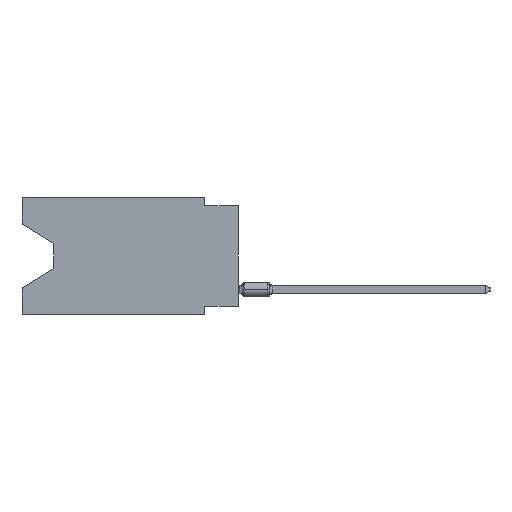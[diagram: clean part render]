
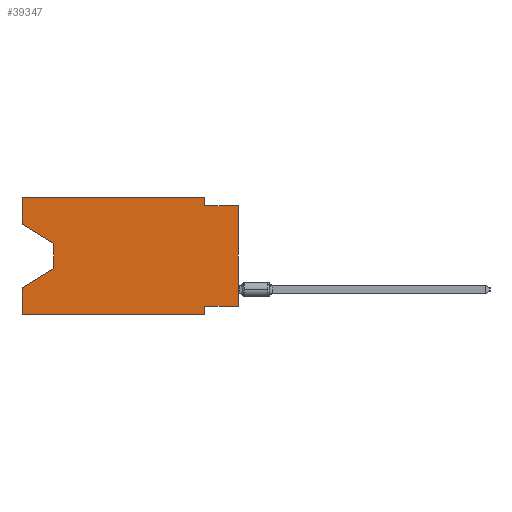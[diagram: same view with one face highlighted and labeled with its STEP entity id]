
A CAD part, left-side view. The second image highlights one B-rep face of the part: STEP entity #39347.
In plain terms, the highlighted planar face has unit normal (-1, 0, 0).
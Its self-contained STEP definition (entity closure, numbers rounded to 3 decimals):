
#670 = LINE ( 'NONE', #19186, #1400 ) ;
#745 = VECTOR ( 'NONE', #2986, 1000. ) ;
#812 = VERTEX_POINT ( 'NONE', #41530 ) ;
#1118 = ORIENTED_EDGE ( 'NONE', *, *, #11759, .T. ) ;
#1400 = VECTOR ( 'NONE', #22766, 1000. ) ;
#2557 = CARTESIAN_POINT ( 'NONE',  ( 0., 2.54, 0. ) ) ;
#2986 = DIRECTION ( 'NONE',  ( 0., 0., 1. ) ) ;
#3231 = CARTESIAN_POINT ( 'NONE',  ( 0., 0., 0. ) ) ;
#3430 = VECTOR ( 'NONE', #35877, 1000. ) ;
#3504 = ORIENTED_EDGE ( 'NONE', *, *, #15011, .T. ) ;
#3566 = VERTEX_POINT ( 'NONE', #45444 ) ;
#5263 = CARTESIAN_POINT ( 'NONE',  ( 0., 16.383, 0. ) ) ;
#5274 = VERTEX_POINT ( 'NONE', #5263 ) ;
#5816 = ORIENTED_EDGE ( 'NONE', *, *, #46398, .F. ) ;
#6011 = ORIENTED_EDGE ( 'NONE', *, *, #12647, .T. ) ;
#6491 = EDGE_CURVE ( 'NONE', #15405, #45929, #42858, .T. ) ;
#6993 = LINE ( 'NONE', #28385, #12425 ) ;
#7243 = LINE ( 'NONE', #25737, #43399 ) ;
#7698 = EDGE_CURVE ( 'NONE', #36288, #3566, #29592, .T. ) ;
#8846 = CARTESIAN_POINT ( 'NONE',  ( 0., 16.383, 0. ) ) ;
#9758 = LINE ( 'NONE', #2557, #27354 ) ;
#10437 = EDGE_CURVE ( 'NONE', #45929, #31728, #40064, .T. ) ;
#10516 = VERTEX_POINT ( 'NONE', #29495 ) ;
#11190 = VECTOR ( 'NONE', #22400, 1000. ) ;
#11759 = EDGE_CURVE ( 'NONE', #15405, #44175, #46711, .T. ) ;
#12163 = VECTOR ( 'NONE', #35338, 1000. ) ;
#12425 = VECTOR ( 'NONE', #20703, 1000. ) ;
#12647 = EDGE_CURVE ( 'NONE', #36288, #31728, #14582, .T. ) ;
#13265 = ORIENTED_EDGE ( 'NONE', *, *, #13916, .F. ) ;
#13916 = EDGE_CURVE ( 'NONE', #23383, #5274, #29414, .T. ) ;
#14513 = VERTEX_POINT ( 'NONE', #23809 ) ;
#14582 = LINE ( 'NONE', #33090, #31527 ) ;
#15011 = EDGE_CURVE ( 'NONE', #14513, #3566, #37028, .T. ) ;
#15405 = VERTEX_POINT ( 'NONE', #15971 ) ;
#15971 = CARTESIAN_POINT ( 'NONE',  ( 0., 0., -8.255 ) ) ;
#16225 = EDGE_CURVE ( 'NONE', #812, #44175, #670, .T. ) ;
#19186 = CARTESIAN_POINT ( 'NONE',  ( 0., 0., -0.635 ) ) ;
#19281 = CARTESIAN_POINT ( 'NONE',  ( 0., 2.54, 0. ) ) ;
#19666 = FACE_OUTER_BOUND ( 'NONE', #25329, .T. ) ;
#20646 = EDGE_CURVE ( 'NONE', #5274, #33728, #27756, .T. ) ;
#20703 = DIRECTION ( 'NONE',  ( 0., 0., -1. ) ) ;
#21094 = ORIENTED_EDGE ( 'NONE', *, *, #10437, .F. ) ;
#22118 = ORIENTED_EDGE ( 'NONE', *, *, #31734, .T. ) ;
#22400 = DIRECTION ( 'NONE',  ( 0., 0., 1. ) ) ;
#22766 = DIRECTION ( 'NONE',  ( 0., -1., 0. ) ) ;
#22799 = CARTESIAN_POINT ( 'NONE',  ( 0., 16.383, -8.89 ) ) ;
#23043 = VECTOR ( 'NONE', #42412, 1000. ) ;
#23383 = VERTEX_POINT ( 'NONE', #42992 ) ;
#23809 = CARTESIAN_POINT ( 'NONE',  ( 0., 13.97, -5.385 ) ) ;
#24850 = CARTESIAN_POINT ( 'NONE',  ( 0., 0., -8.255 ) ) ;
#25329 = EDGE_LOOP ( 'NONE', ( #22118, #37161, #3504, #45902, #6011, #21094, #42938, #1118, #45962, #5816, #39247, #13265 ) ) ;
#25737 = CARTESIAN_POINT ( 'NONE',  ( 0., 16.383, -2.038 ) ) ;
#25791 = CARTESIAN_POINT ( 'NONE',  ( 0., 16.383, 0. ) ) ;
#26452 = CARTESIAN_POINT ( 'NONE',  ( 0., 13.97, -5.385 ) ) ;
#27354 = VECTOR ( 'NONE', #27809, 1000. ) ;
#27397 = VECTOR ( 'NONE', #37972, 1000. ) ;
#27425 = CARTESIAN_POINT ( 'NONE',  ( 0., 0., -0.635 ) ) ;
#27655 = DIRECTION ( 'NONE',  ( 0., -1., 0. ) ) ;
#27756 = LINE ( 'NONE', #34939, #23043 ) ;
#27809 = DIRECTION ( 'NONE',  ( 0., 0., -1. ) ) ;
#28018 = EDGE_CURVE ( 'NONE', #10516, #14513, #6993, .T. ) ;
#28385 = CARTESIAN_POINT ( 'NONE',  ( 0., 13.97, -3.505 ) ) ;
#29414 = LINE ( 'NONE', #25791, #33573 ) ;
#29495 = CARTESIAN_POINT ( 'NONE',  ( 0., 13.97, -3.505 ) ) ;
#29592 = LINE ( 'NONE', #33682, #11190 ) ;
#31527 = VECTOR ( 'NONE', #27655, 1000. ) ;
#31728 = VERTEX_POINT ( 'NONE', #43504 ) ;
#31734 = EDGE_CURVE ( 'NONE', #23383, #10516, #7243, .T. ) ;
#32162 = CARTESIAN_POINT ( 'NONE',  ( 0., 2.54, -8.255 ) ) ;
#33090 = CARTESIAN_POINT ( 'NONE',  ( 0., 16.383, -8.89 ) ) ;
#33573 = VECTOR ( 'NONE', #34193, 1000. ) ;
#33682 = CARTESIAN_POINT ( 'NONE',  ( 0., 16.383, 0. ) ) ;
#33728 = VERTEX_POINT ( 'NONE', #19281 ) ;
#34193 = DIRECTION ( 'NONE',  ( 0., 0., 1. ) ) ;
#34939 = CARTESIAN_POINT ( 'NONE',  ( 0., 16.383, 0. ) ) ;
#35338 = DIRECTION ( 'NONE',  ( 0., 0., -1. ) ) ;
#35877 = DIRECTION ( 'NONE',  ( 0., 1., 0. ) ) ;
#36288 = VERTEX_POINT ( 'NONE', #22799 ) ;
#37028 = LINE ( 'NONE', #26452, #27397 ) ;
#37161 = ORIENTED_EDGE ( 'NONE', *, *, #28018, .T. ) ;
#37972 = DIRECTION ( 'NONE',  ( 0., 0.855, -0.519 ) ) ;
#39247 = ORIENTED_EDGE ( 'NONE', *, *, #20646, .F. ) ;
#39251 = AXIS2_PLACEMENT_3D ( 'NONE', #8846, #43336, #47426 ) ;
#39347 = ADVANCED_FACE ( 'NONE', ( #19666 ), #41773, .F. ) ;
#40064 = LINE ( 'NONE', #46605, #12163 ) ;
#40382 = DIRECTION ( 'NONE',  ( 0., -0.855, -0.519 ) ) ;
#41530 = CARTESIAN_POINT ( 'NONE',  ( 0., 2.54, -0.635 ) ) ;
#41773 = PLANE ( 'NONE',  #39251 ) ;
#42412 = DIRECTION ( 'NONE',  ( 0., -1., 0. ) ) ;
#42858 = LINE ( 'NONE', #24850, #3430 ) ;
#42938 = ORIENTED_EDGE ( 'NONE', *, *, #6491, .F. ) ;
#42992 = CARTESIAN_POINT ( 'NONE',  ( 0., 16.383, -2.038 ) ) ;
#43336 = DIRECTION ( 'NONE',  ( 1., 0., 0. ) ) ;
#43399 = VECTOR ( 'NONE', #40382, 1000. ) ;
#43504 = CARTESIAN_POINT ( 'NONE',  ( 0., 2.54, -8.89 ) ) ;
#44175 = VERTEX_POINT ( 'NONE', #27425 ) ;
#45444 = CARTESIAN_POINT ( 'NONE',  ( 0., 16.383, -6.852 ) ) ;
#45902 = ORIENTED_EDGE ( 'NONE', *, *, #7698, .F. ) ;
#45929 = VERTEX_POINT ( 'NONE', #32162 ) ;
#45962 = ORIENTED_EDGE ( 'NONE', *, *, #16225, .F. ) ;
#46398 = EDGE_CURVE ( 'NONE', #33728, #812, #9758, .T. ) ;
#46605 = CARTESIAN_POINT ( 'NONE',  ( 0., 2.54, -8.89 ) ) ;
#46711 = LINE ( 'NONE', #3231, #745 ) ;
#47426 = DIRECTION ( 'NONE',  ( 0., 0., -1. ) ) ;
